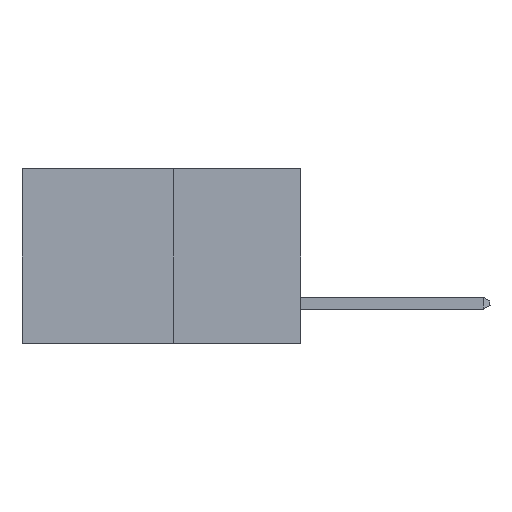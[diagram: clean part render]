
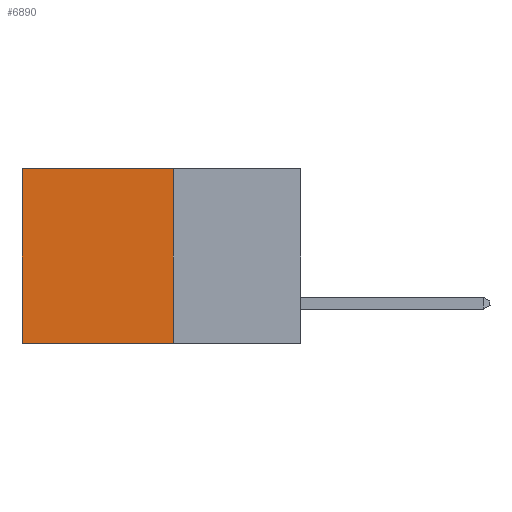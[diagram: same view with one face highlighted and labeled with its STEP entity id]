
A CAD part, left-side view. The second image highlights one B-rep face of the part: STEP entity #6890.
In plain terms, the highlighted planar face has unit normal (-1, 0, 0).
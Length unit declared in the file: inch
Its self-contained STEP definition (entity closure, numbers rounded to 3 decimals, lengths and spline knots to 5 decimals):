
#126 = VERTEX_POINT ( 'NONE', #10757 ) ;
#932 = ORIENTED_EDGE ( 'NONE', *, *, #15798, .F. ) ;
#1259 = DIRECTION ( 'NONE',  ( 0., 0., -1. ) ) ;
#1492 = VECTOR ( 'NONE', #10198, 39.37008 ) ;
#2317 = EDGE_LOOP ( 'NONE', ( #9378, #6870, #932, #14035 ) ) ;
#2632 = CARTESIAN_POINT ( 'NONE',  ( 0.277, 0.27, 0. ) ) ;
#3196 = CARTESIAN_POINT ( 'NONE',  ( 0.277, 0.27, -0.37 ) ) ;
#3597 = LINE ( 'NONE', #9133, #12101 ) ;
#3884 = DIRECTION ( 'NONE',  ( 0., 1., 0. ) ) ;
#4754 = CARTESIAN_POINT ( 'NONE',  ( 0.277, 0.59, -0.37 ) ) ;
#5217 = FACE_OUTER_BOUND ( 'NONE', #2317, .T. ) ;
#5531 = LINE ( 'NONE', #9646, #13548 ) ;
#6870 = ORIENTED_EDGE ( 'NONE', *, *, #10834, .F. ) ;
#6890 = ADVANCED_FACE ( 'NONE', ( #5217 ), #11127, .F. ) ;
#8610 = CARTESIAN_POINT ( 'NONE',  ( 0.277, 0.27, 0. ) ) ;
#9133 = CARTESIAN_POINT ( 'NONE',  ( 0.277, 0.59, -0.37 ) ) ;
#9378 = ORIENTED_EDGE ( 'NONE', *, *, #15074, .T. ) ;
#9530 = VECTOR ( 'NONE', #3884, 39.37008 ) ;
#9646 = CARTESIAN_POINT ( 'NONE',  ( 0.277, 0.27, -0.37 ) ) ;
#9666 = VERTEX_POINT ( 'NONE', #2632 ) ;
#10198 = DIRECTION ( 'NONE',  ( 0., 1., 0. ) ) ;
#10757 = CARTESIAN_POINT ( 'NONE',  ( 0.277, 0.59, 0. ) ) ;
#10834 = EDGE_CURVE ( 'NONE', #20499, #12704, #18531, .T. ) ;
#10982 = DIRECTION ( 'NONE',  ( 0., 0., -1. ) ) ;
#11009 = DIRECTION ( 'NONE',  ( 1., 0., 0. ) ) ;
#11060 = CARTESIAN_POINT ( 'NONE',  ( 0.277, 0.27, -0.37 ) ) ;
#11127 = PLANE ( 'NONE',  #19701 ) ;
#11289 = DIRECTION ( 'NONE',  ( 0., 0., -1. ) ) ;
#11813 = CARTESIAN_POINT ( 'NONE',  ( 0.277, 0.27, -0.37 ) ) ;
#12101 = VECTOR ( 'NONE', #1259, 39.37008 ) ;
#12704 = VERTEX_POINT ( 'NONE', #4754 ) ;
#13548 = VECTOR ( 'NONE', #11289, 39.37008 ) ;
#14035 = ORIENTED_EDGE ( 'NONE', *, *, #20154, .T. ) ;
#15074 = EDGE_CURVE ( 'NONE', #126, #12704, #3597, .T. ) ;
#15798 = EDGE_CURVE ( 'NONE', #9666, #20499, #5531, .T. ) ;
#18531 = LINE ( 'NONE', #11813, #9530 ) ;
#18850 = LINE ( 'NONE', #8610, #1492 ) ;
#19701 = AXIS2_PLACEMENT_3D ( 'NONE', #11060, #11009, #10982 ) ;
#20154 = EDGE_CURVE ( 'NONE', #9666, #126, #18850, .T. ) ;
#20499 = VERTEX_POINT ( 'NONE', #3196 ) ;
